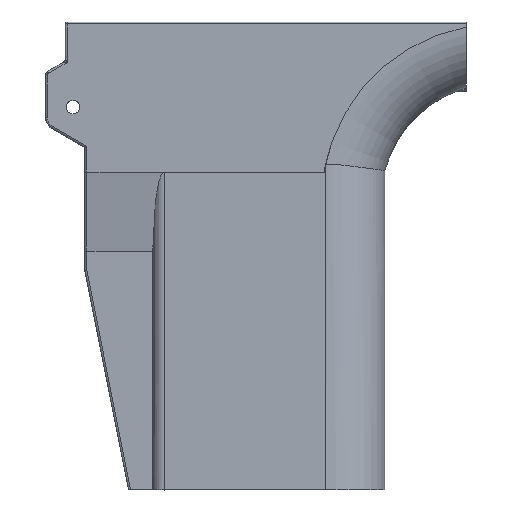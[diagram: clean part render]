
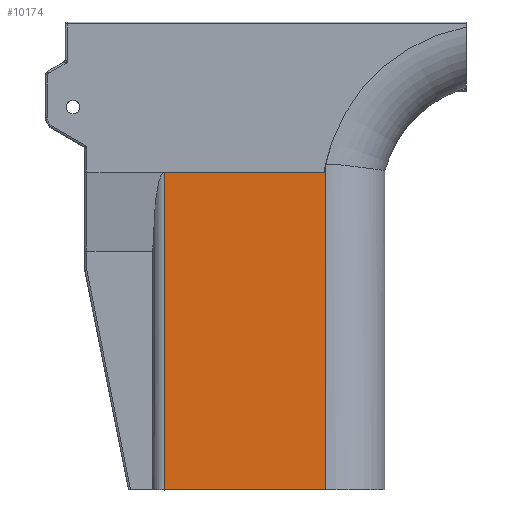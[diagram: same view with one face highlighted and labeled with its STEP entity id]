
A CAD part, top view. The second image highlights one B-rep face of the part: STEP entity #10174.
In plain terms, the highlighted planar face has unit normal (0, 0, 1).
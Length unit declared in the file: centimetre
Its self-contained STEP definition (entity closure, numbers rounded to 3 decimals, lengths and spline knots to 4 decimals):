
#304=PLANE($,#10876);
#655=FACE_OUTER_BOUND($,#1298,.T.);
#1298=EDGE_LOOP($,(#7102,#7103,#7104,#7105,#7106,#7107,#7108,#7109));
#1989=CIRCLE($,#10877,4.4939);
#2341=LINE($,#15065,#3329);
#2398=LINE($,#15298,#3386);
#2399=LINE($,#15300,#3387);
#2404=LINE($,#15317,#3392);
#2426=LINE($,#15429,#3414);
#2427=LINE($,#15430,#3415);
#2428=LINE($,#15433,#3416);
#3329=VECTOR($,#11881,8.2388);
#3386=VECTOR($,#12028,0.18);
#3387=VECTOR($,#12029,3.9);
#3392=VECTOR($,#12044,8.0449);
#3414=VECTOR($,#12134,4.0366);
#3415=VECTOR($,#12135,0.0001);
#3416=VECTOR($,#12138,0.0062);
#4402=VERTEX_POINT($,#15059);
#4403=VERTEX_POINT($,#15064);
#4483=VERTEX_POINT($,#15297);
#4484=VERTEX_POINT($,#15299);
#4491=VERTEX_POINT($,#15314);
#4515=VERTEX_POINT($,#15427);
#4516=VERTEX_POINT($,#15428);
#4517=VERTEX_POINT($,#15431);
#5339=EDGE_CURVE($,#4402,#4403,#2341,.T.);
#5434=EDGE_CURVE($,#4483,#4403,#2398,.F.);
#5435=EDGE_CURVE($,#4484,#4483,#2399,.F.);
#5444=EDGE_CURVE($,#4484,#4491,#2404,.T.);
#5486=EDGE_CURVE($,#4515,#4516,#2426,.T.);
#5487=EDGE_CURVE($,#4491,#4515,#2427,.F.);
#5488=EDGE_CURVE($,#4517,#4402,#1989,.T.);
#5489=EDGE_CURVE($,#4516,#4517,#2428,.T.);
#7102=ORIENTED_EDGE($,*,*,#5486,.F.);
#7103=ORIENTED_EDGE($,*,*,#5487,.F.);
#7104=ORIENTED_EDGE($,*,*,#5444,.F.);
#7105=ORIENTED_EDGE($,*,*,#5435,.T.);
#7106=ORIENTED_EDGE($,*,*,#5434,.T.);
#7107=ORIENTED_EDGE($,*,*,#5339,.F.);
#7108=ORIENTED_EDGE($,*,*,#5488,.F.);
#7109=ORIENTED_EDGE($,*,*,#5489,.F.);
#10174=ADVANCED_FACE($,(#655),#304,.F.);
#10876=AXIS2_PLACEMENT_3D($,#15426,#12132,#12133);
#10877=AXIS2_PLACEMENT_3D($,#15432,#12136,#12137);
#11881=DIRECTION($,(0.,-1.,0.));
#12028=DIRECTION($,(-1.,0.,0.));
#12029=DIRECTION($,(-1.,0.,0.));
#12044=DIRECTION($,(0.,1.,0.));
#12132=DIRECTION('center_axis',(0.,0.,
-1.));
#12133=DIRECTION('ref_axis',(0.,-1.,0.));
#12134=DIRECTION($,(1.,0.,0.));
#12135=DIRECTION($,(0.,-0.989,-0.148));
#12136=DIRECTION('center_axis',(0.,0.,
-1.));
#12137=DIRECTION('ref_axis',(-1.,0.,0.));
#12138=DIRECTION($,(1.,0.,0.));
#15059=CARTESIAN_POINT('',(-2.3936,-4.4352,2.));
#15064=CARTESIAN_POINT('',(-2.3936,-12.674,2.));
#15065=CARTESIAN_POINT($,(-2.3936,-12.674,2.));
#15297=CARTESIAN_POINT('',(-2.5736,-12.674,2.));
#15298=CARTESIAN_POINT($,(-4.4752,-12.674,2.));
#15299=CARTESIAN_POINT('',(-6.4736,-12.674,2.));
#15300=CARTESIAN_POINT($,(-4.4752,-12.674,2.));
#15314=CARTESIAN_POINT('',(-6.4736,-4.6291,2.));
#15317=CARTESIAN_POINT($,(-6.4736,-12.4244,2.));
#15426=CARTESIAN_POINT('Origin',(-4.4736,-12.4244,2.));
#15427=CARTESIAN_POINT('',(-6.4736,-4.629,2.));
#15428=CARTESIAN_POINT('',(-2.4371,-4.629,2.));
#15429=CARTESIAN_POINT($,(-2.964,-4.629,2.));
#15430=CARTESIAN_POINT($,(-6.4736,-5.7518,1.8316));
#15431=CARTESIAN_POINT('',(-2.4308,-4.629,2.));
#15432=CARTESIAN_POINT('Origin',(2.,-5.379,2.));
#15433=CARTESIAN_POINT($,(-2.964,-4.629,2.));
